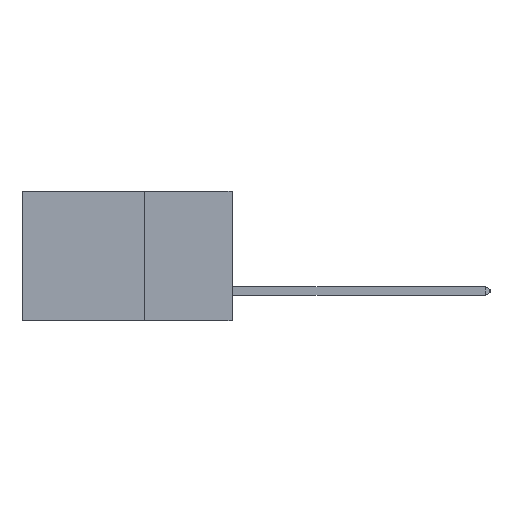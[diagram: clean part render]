
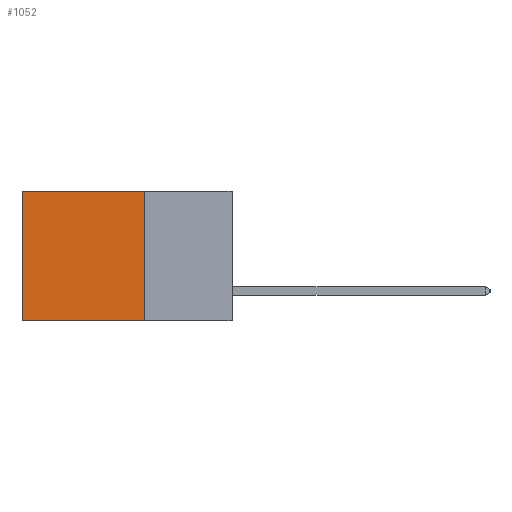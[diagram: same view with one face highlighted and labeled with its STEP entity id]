
A CAD part, left-side view. The second image highlights one B-rep face of the part: STEP entity #1052.
In plain terms, the highlighted planar face has unit normal (-1, 0, 0).
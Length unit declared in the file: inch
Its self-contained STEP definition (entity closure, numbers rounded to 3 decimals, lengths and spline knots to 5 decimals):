
#19 = EDGE_CURVE ( 'NONE', #3907, #6745, #17981, .T. ) ;
#305 = ORIENTED_EDGE ( 'NONE', *, *, #5933, .F. ) ;
#1052 = ADVANCED_FACE ( 'NONE', ( #13912 ), #12008, .F. ) ;
#1141 = VECTOR ( 'NONE', #12069, 39.37008 ) ;
#2065 = CARTESIAN_POINT ( 'NONE',  ( 0.2875, 0.25, 0. ) ) ;
#2131 = VECTOR ( 'NONE', #6831, 39.37008 ) ;
#3691 = CARTESIAN_POINT ( 'NONE',  ( 0.2875, 0.25, 0. ) ) ;
#3907 = VERTEX_POINT ( 'NONE', #2065 ) ;
#4276 = ORIENTED_EDGE ( 'NONE', *, *, #9602, .T. ) ;
#5222 = EDGE_CURVE ( 'NONE', #6218, #9104, #12913, .T. ) ;
#5433 = AXIS2_PLACEMENT_3D ( 'NONE', #12213, #11964, #11776 ) ;
#5440 = VECTOR ( 'NONE', #16305, 39.37008 ) ;
#5933 = EDGE_CURVE ( 'NONE', #6745, #9104, #16531, .T. ) ;
#6218 = VERTEX_POINT ( 'NONE', #17083 ) ;
#6745 = VERTEX_POINT ( 'NONE', #9907 ) ;
#6831 = DIRECTION ( 'NONE',  ( 0., 1., 0. ) ) ;
#7095 = ORIENTED_EDGE ( 'NONE', *, *, #19, .F. ) ;
#7958 = CARTESIAN_POINT ( 'NONE',  ( 0.2875, 0.6, 0. ) ) ;
#8121 = LINE ( 'NONE', #3691, #1141 ) ;
#8207 = DIRECTION ( 'NONE',  ( 0., 0., -1. ) ) ;
#8227 = CARTESIAN_POINT ( 'NONE',  ( 0.2875, 0.6, -0.37 ) ) ;
#8829 = CARTESIAN_POINT ( 'NONE',  ( 0.2875, 0.25, 0. ) ) ;
#9104 = VERTEX_POINT ( 'NONE', #8227 ) ;
#9602 = EDGE_CURVE ( 'NONE', #3907, #6218, #8121, .T. ) ;
#9907 = CARTESIAN_POINT ( 'NONE',  ( 0.2875, 0.25, -0.37 ) ) ;
#11776 = DIRECTION ( 'NONE',  ( 0., 0., -1. ) ) ;
#11964 = DIRECTION ( 'NONE',  ( 1., 0., 0. ) ) ;
#12008 = PLANE ( 'NONE',  #5433 ) ;
#12069 = DIRECTION ( 'NONE',  ( 0., 1., 0. ) ) ;
#12213 = CARTESIAN_POINT ( 'NONE',  ( 0.2875, 0.25, 0. ) ) ;
#12913 = LINE ( 'NONE', #7958, #5440 ) ;
#13912 = FACE_OUTER_BOUND ( 'NONE', #16641, .T. ) ;
#13929 = VECTOR ( 'NONE', #8207, 39.37008 ) ;
#16199 = ORIENTED_EDGE ( 'NONE', *, *, #5222, .T. ) ;
#16305 = DIRECTION ( 'NONE',  ( 0., 0., -1. ) ) ;
#16531 = LINE ( 'NONE', #17940, #2131 ) ;
#16641 = EDGE_LOOP ( 'NONE', ( #16199, #305, #7095, #4276 ) ) ;
#17083 = CARTESIAN_POINT ( 'NONE',  ( 0.2875, 0.6, 0. ) ) ;
#17940 = CARTESIAN_POINT ( 'NONE',  ( 0.2875, 0.25, -0.37 ) ) ;
#17981 = LINE ( 'NONE', #8829, #13929 ) ;
